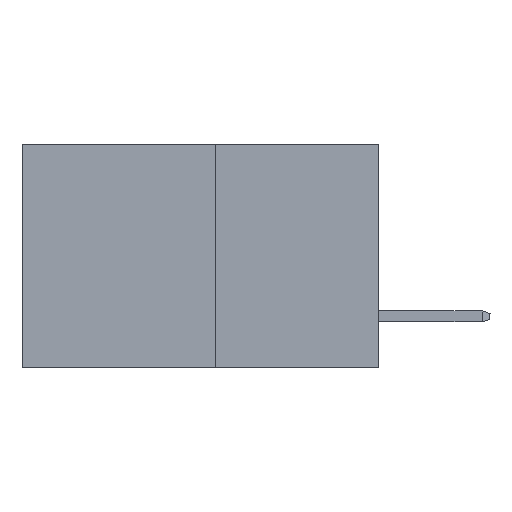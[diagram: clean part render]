
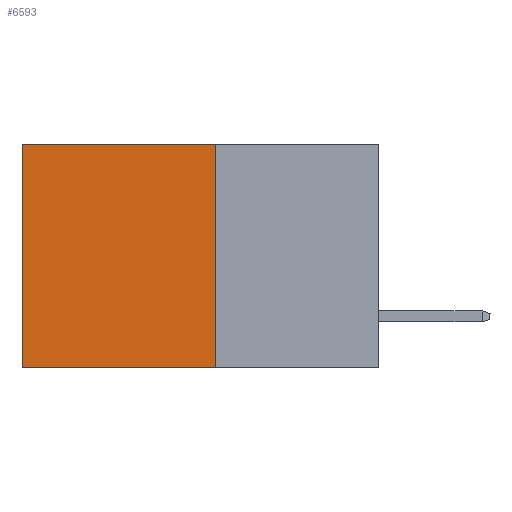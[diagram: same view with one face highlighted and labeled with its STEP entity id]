
A CAD part, left-side view. The second image highlights one B-rep face of the part: STEP entity #6593.
In plain terms, the highlighted planar face has unit normal (-1, 0, 0).
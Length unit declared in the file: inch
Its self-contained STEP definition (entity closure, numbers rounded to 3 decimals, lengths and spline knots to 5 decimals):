
#3 = VERTEX_POINT ( 'NONE', #209 ) ;
#16 = EDGE_CURVE ( 'NONE', #3238, #3, #977, .T. ) ;
#26 = CARTESIAN_POINT ( 'NONE',  ( 0.277, 0.27, 0. ) ) ;
#31 = CARTESIAN_POINT ( 'NONE',  ( 0.277, 0.27, -0.37 ) ) ;
#209 = CARTESIAN_POINT ( 'NONE',  ( 0.277, 0.59, 0. ) ) ;
#956 = DIRECTION ( 'NONE',  ( 0., 0., -1. ) ) ;
#977 = LINE ( 'NONE', #26, #8388 ) ;
#979 = EDGE_CURVE ( 'NONE', #3, #6592, #6854, .T. ) ;
#2019 = EDGE_CURVE ( 'NONE', #3238, #4450, #6416, .T. ) ;
#2426 = EDGE_LOOP ( 'NONE', ( #4722, #3832, #3010, #6330 ) ) ;
#2634 = DIRECTION ( 'NONE',  ( 0., 1., 0. ) ) ;
#2671 = CARTESIAN_POINT ( 'NONE',  ( 0.277, 0.27, -0.37 ) ) ;
#3010 = ORIENTED_EDGE ( 'NONE', *, *, #2019, .F. ) ;
#3238 = VERTEX_POINT ( 'NONE', #8084 ) ;
#3832 = ORIENTED_EDGE ( 'NONE', *, *, #4237, .F. ) ;
#4237 = EDGE_CURVE ( 'NONE', #4450, #6592, #5209, .T. ) ;
#4450 = VERTEX_POINT ( 'NONE', #31 ) ;
#4562 = VECTOR ( 'NONE', #6437, 39.37008 ) ;
#4722 = ORIENTED_EDGE ( 'NONE', *, *, #979, .T. ) ;
#5090 = VECTOR ( 'NONE', #956, 39.37008 ) ;
#5209 = LINE ( 'NONE', #2671, #7174 ) ;
#5420 = DIRECTION ( 'NONE',  ( 0., 0., -1. ) ) ;
#5428 = DIRECTION ( 'NONE',  ( 1., 0., 0. ) ) ;
#5447 = CARTESIAN_POINT ( 'NONE',  ( 0.277, 0.27, -0.37 ) ) ;
#5477 = PLANE ( 'NONE',  #7359 ) ;
#5520 = CARTESIAN_POINT ( 'NONE',  ( 0.277, 0.59, -0.37 ) ) ;
#6327 = CARTESIAN_POINT ( 'NONE',  ( 0.277, 0.27, -0.37 ) ) ;
#6330 = ORIENTED_EDGE ( 'NONE', *, *, #16, .T. ) ;
#6410 = DIRECTION ( 'NONE',  ( 0., 1., 0. ) ) ;
#6416 = LINE ( 'NONE', #6327, #4562 ) ;
#6437 = DIRECTION ( 'NONE',  ( 0., 0., -1. ) ) ;
#6592 = VERTEX_POINT ( 'NONE', #5520 ) ;
#6593 = ADVANCED_FACE ( 'NONE', ( #7816 ), #5477, .F. ) ;
#6836 = CARTESIAN_POINT ( 'NONE',  ( 0.277, 0.59, -0.37 ) ) ;
#6854 = LINE ( 'NONE', #6836, #5090 ) ;
#7174 = VECTOR ( 'NONE', #2634, 39.37008 ) ;
#7359 = AXIS2_PLACEMENT_3D ( 'NONE', #5447, #5428, #5420 ) ;
#7816 = FACE_OUTER_BOUND ( 'NONE', #2426, .T. ) ;
#8084 = CARTESIAN_POINT ( 'NONE',  ( 0.277, 0.27, 0. ) ) ;
#8388 = VECTOR ( 'NONE', #6410, 39.37008 ) ;
